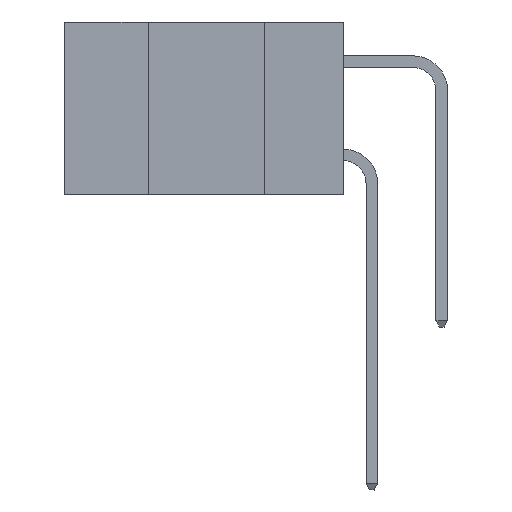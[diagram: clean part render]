
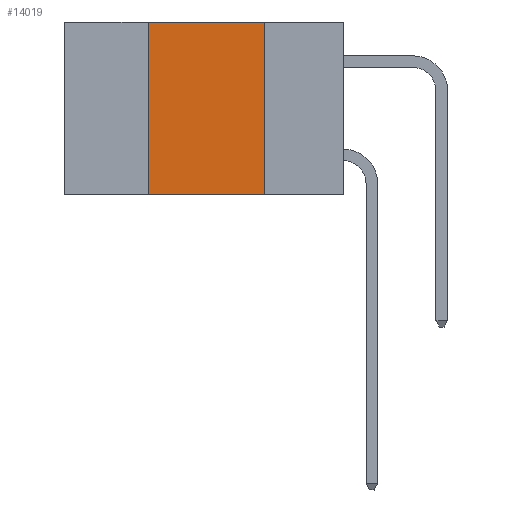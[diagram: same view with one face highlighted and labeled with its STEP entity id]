
A CAD part, left-side view. The second image highlights one B-rep face of the part: STEP entity #14019.
In plain terms, the highlighted planar face has unit normal (-1, 0, 0).
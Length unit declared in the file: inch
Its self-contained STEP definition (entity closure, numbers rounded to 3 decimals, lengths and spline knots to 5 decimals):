
#234 = EDGE_CURVE ( 'NONE', #17359, #18582, #19743, .T. ) ;
#2096 = FACE_OUTER_BOUND ( 'NONE', #22968, .T. ) ;
#2742 = ORIENTED_EDGE ( 'NONE', *, *, #3624, .T. ) ;
#3624 = EDGE_CURVE ( 'NONE', #17359, #7249, #7784, .T. ) ;
#4093 = DIRECTION ( 'NONE',  ( 1., 0., 0. ) ) ;
#6316 = DIRECTION ( 'NONE',  ( 0., 0., 1. ) ) ;
#6760 = VECTOR ( 'NONE', #9078, 39.37008 ) ;
#6769 = ORIENTED_EDGE ( 'NONE', *, *, #12632, .F. ) ;
#7151 = ORIENTED_EDGE ( 'NONE', *, *, #11968, .F. ) ;
#7249 = VERTEX_POINT ( 'NONE', #24999 ) ;
#7784 = LINE ( 'NONE', #18129, #19252 ) ;
#8273 = DIRECTION ( 'NONE',  ( 0., 0., -1. ) ) ;
#8619 = ORIENTED_EDGE ( 'NONE', *, *, #234, .F. ) ;
#9078 = DIRECTION ( 'NONE',  ( 0., -1., 0. ) ) ;
#11056 = CARTESIAN_POINT ( 'NONE',  ( 0., 0.17, 0. ) ) ;
#11215 = LINE ( 'NONE', #22110, #6760 ) ;
#11968 = EDGE_CURVE ( 'NONE', #18582, #24357, #11215, .T. ) ;
#12632 = EDGE_CURVE ( 'NONE', #24357, #7249, #19041, .T. ) ;
#13502 = VECTOR ( 'NONE', #8273, 39.37008 ) ;
#13982 = CARTESIAN_POINT ( 'NONE',  ( 0., 0.42, -0.37 ) ) ;
#14019 = ADVANCED_FACE ( 'NONE', ( #2096 ), #17259, .F. ) ;
#15869 = DIRECTION ( 'NONE',  ( 0., -1., 0. ) ) ;
#17259 = PLANE ( 'NONE',  #26068 ) ;
#17359 = VERTEX_POINT ( 'NONE', #13982 ) ;
#17623 = CARTESIAN_POINT ( 'NONE',  ( 0., 0.42, -0.37 ) ) ;
#18129 = CARTESIAN_POINT ( 'NONE',  ( 0., 0.6, -0.37 ) ) ;
#18582 = VERTEX_POINT ( 'NONE', #20743 ) ;
#19041 = LINE ( 'NONE', #27667, #13502 ) ;
#19252 = VECTOR ( 'NONE', #15869, 39.37008 ) ;
#19743 = LINE ( 'NONE', #17623, #23223 ) ;
#20743 = CARTESIAN_POINT ( 'NONE',  ( 0., 0.42, 0. ) ) ;
#22110 = CARTESIAN_POINT ( 'NONE',  ( 0., 0.6, 0. ) ) ;
#22968 = EDGE_LOOP ( 'NONE', ( #6769, #7151, #8619, #2742 ) ) ;
#23223 = VECTOR ( 'NONE', #6316, 39.37008 ) ;
#24357 = VERTEX_POINT ( 'NONE', #11056 ) ;
#24999 = CARTESIAN_POINT ( 'NONE',  ( 0., 0.17, -0.37 ) ) ;
#25597 = CARTESIAN_POINT ( 'NONE',  ( 0., 0.6, 0. ) ) ;
#25750 = DIRECTION ( 'NONE',  ( 0., 0., -1. ) ) ;
#26068 = AXIS2_PLACEMENT_3D ( 'NONE', #25597, #4093, #25750 ) ;
#27667 = CARTESIAN_POINT ( 'NONE',  ( 0., 0.17, -0.37 ) ) ;
